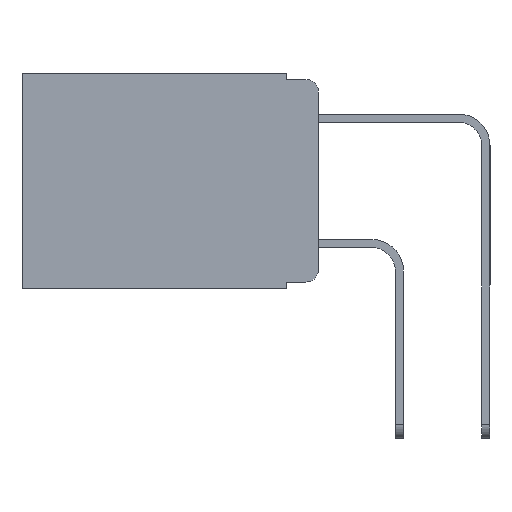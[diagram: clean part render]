
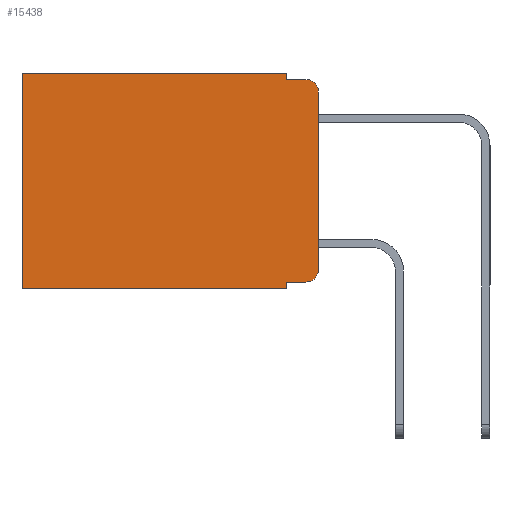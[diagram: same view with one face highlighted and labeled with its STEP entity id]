
A CAD part, left-side view. The second image highlights one B-rep face of the part: STEP entity #15438.
In plain terms, the highlighted planar face has unit normal (-1, 0, 0).
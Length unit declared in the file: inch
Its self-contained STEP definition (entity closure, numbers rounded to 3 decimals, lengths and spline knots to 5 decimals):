
#129 = CARTESIAN_POINT ( 'NONE',  ( 0.298, 0.473, 0. ) ) ;
#816 = VERTEX_POINT ( 'NONE', #3962 ) ;
#822 = DIRECTION ( 'NONE',  ( 0., 1., 0. ) ) ;
#897 = CARTESIAN_POINT ( 'NONE',  ( 0.298, 0., -0.343 ) ) ;
#1227 = ORIENTED_EDGE ( 'NONE', *, *, #1581, .T. ) ;
#1581 = EDGE_CURVE ( 'NONE', #16768, #816, #11439, .T. ) ;
#1775 = VECTOR ( 'NONE', #6155, 39.37008 ) ;
#1896 = VERTEX_POINT ( 'NONE', #14974 ) ;
#2503 = CARTESIAN_POINT ( 'NONE',  ( 0.298, 0.02, -0.03 ) ) ;
#2618 = VECTOR ( 'NONE', #7632, 39.37008 ) ;
#2688 = EDGE_CURVE ( 'NONE', #15392, #16768, #8847, .T. ) ;
#3005 = ORIENTED_EDGE ( 'NONE', *, *, #16992, .T. ) ;
#3034 = DIRECTION ( 'NONE',  ( 0., -1., 0. ) ) ;
#3763 = EDGE_CURVE ( 'NONE', #15392, #4194, #6385, .T. ) ;
#3962 = CARTESIAN_POINT ( 'NONE',  ( 0.298, 0., -0.313 ) ) ;
#3990 = ORIENTED_EDGE ( 'NONE', *, *, #2688, .T. ) ;
#3991 = AXIS2_PLACEMENT_3D ( 'NONE', #16512, #12750, #4978 ) ;
#4094 = DIRECTION ( 'NONE',  ( 0., 0., -1. ) ) ;
#4194 = VERTEX_POINT ( 'NONE', #15497 ) ;
#4494 = LINE ( 'NONE', #129, #5742 ) ;
#4729 = EDGE_CURVE ( 'NONE', #1896, #7967, #4494, .T. ) ;
#4978 = DIRECTION ( 'NONE',  ( 0., 0., -1. ) ) ;
#5184 = AXIS2_PLACEMENT_3D ( 'NONE', #2503, #11911, #4094 ) ;
#5299 = LINE ( 'NONE', #7913, #15559 ) ;
#5421 = DIRECTION ( 'NONE',  ( 0., 0., -1. ) ) ;
#5434 = VECTOR ( 'NONE', #3034, 39.37008 ) ;
#5614 = EDGE_CURVE ( 'NONE', #13787, #12726, #11580, .T. ) ;
#5742 = VECTOR ( 'NONE', #8728, 39.37008 ) ;
#6155 = DIRECTION ( 'NONE',  ( 0., 1., 0. ) ) ;
#6385 = LINE ( 'NONE', #15324, #2618 ) ;
#6475 = EDGE_CURVE ( 'NONE', #12726, #7217, #5299, .T. ) ;
#6719 = ORIENTED_EDGE ( 'NONE', *, *, #5614, .F. ) ;
#6771 = CARTESIAN_POINT ( 'NONE',  ( 0.298, 0.02, -0.313 ) ) ;
#7217 = VERTEX_POINT ( 'NONE', #14213 ) ;
#7240 = DIRECTION ( 'NONE',  ( 0., 0., -1. ) ) ;
#7342 = EDGE_CURVE ( 'NONE', #14983, #7217, #13964, .T. ) ;
#7632 = DIRECTION ( 'NONE',  ( 0., 0., -1. ) ) ;
#7913 = CARTESIAN_POINT ( 'NONE',  ( 0.298, 0.051, -0.01 ) ) ;
#7914 = ORIENTED_EDGE ( 'NONE', *, *, #3763, .F. ) ;
#7967 = VERTEX_POINT ( 'NONE', #10628 ) ;
#8108 = EDGE_LOOP ( 'NONE', ( #8900, #16126, #12771, #6719, #3005, #17295, #10115, #7914, #3990, #1227 ) ) ;
#8112 = CARTESIAN_POINT ( 'NONE',  ( 0.298, 0., -0.03 ) ) ;
#8404 = CARTESIAN_POINT ( 'NONE',  ( 0.298, 0.051, -0.333 ) ) ;
#8728 = DIRECTION ( 'NONE',  ( 0., 0., -1. ) ) ;
#8738 = EDGE_CURVE ( 'NONE', #4194, #7967, #13729, .T. ) ;
#8824 = PLANE ( 'NONE',  #3991 ) ;
#8847 = LINE ( 'NONE', #8404, #5434 ) ;
#8900 = ORIENTED_EDGE ( 'NONE', *, *, #9059, .F. ) ;
#9059 = EDGE_CURVE ( 'NONE', #14983, #816, #16663, .T. ) ;
#10014 = CARTESIAN_POINT ( 'NONE',  ( 0.298, 0.051, -0.333 ) ) ;
#10115 = ORIENTED_EDGE ( 'NONE', *, *, #8738, .F. ) ;
#10628 = CARTESIAN_POINT ( 'NONE',  ( 0.298, 0.473, -0.343 ) ) ;
#10680 = VECTOR ( 'NONE', #822, 39.37008 ) ;
#11319 = CARTESIAN_POINT ( 'NONE',  ( 0.298, 0.051, -0.01 ) ) ;
#11350 = CARTESIAN_POINT ( 'NONE',  ( 0.298, 0., 0. ) ) ;
#11439 = CIRCLE ( 'NONE', #14627, 0.02 ) ;
#11580 = LINE ( 'NONE', #15345, #14593 ) ;
#11803 = CARTESIAN_POINT ( 'NONE',  ( 0.298, 0.051, 0. ) ) ;
#11911 = DIRECTION ( 'NONE',  ( -1., 0., 0. ) ) ;
#12726 = VERTEX_POINT ( 'NONE', #11319 ) ;
#12750 = DIRECTION ( 'NONE',  ( 1., 0., 0. ) ) ;
#12771 = ORIENTED_EDGE ( 'NONE', *, *, #6475, .F. ) ;
#12915 = VECTOR ( 'NONE', #7240, 39.37008 ) ;
#13032 = DIRECTION ( 'NONE',  ( -1., 0., 0. ) ) ;
#13127 = DIRECTION ( 'NONE',  ( 0., -1., 0. ) ) ;
#13729 = LINE ( 'NONE', #897, #10680 ) ;
#13787 = VERTEX_POINT ( 'NONE', #11803 ) ;
#13815 = LINE ( 'NONE', #11350, #1775 ) ;
#13964 = CIRCLE ( 'NONE', #5184, 0.02 ) ;
#14081 = DIRECTION ( 'NONE',  ( 0., 0., -1. ) ) ;
#14213 = CARTESIAN_POINT ( 'NONE',  ( 0.298, 0.02, -0.01 ) ) ;
#14593 = VECTOR ( 'NONE', #14081, 39.37008 ) ;
#14627 = AXIS2_PLACEMENT_3D ( 'NONE', #6771, #13032, #5421 ) ;
#14935 = CARTESIAN_POINT ( 'NONE',  ( 0.298, 0.02, -0.333 ) ) ;
#14974 = CARTESIAN_POINT ( 'NONE',  ( 0.298, 0.473, 0. ) ) ;
#14983 = VERTEX_POINT ( 'NONE', #8112 ) ;
#15033 = FACE_OUTER_BOUND ( 'NONE', #8108, .T. ) ;
#15324 = CARTESIAN_POINT ( 'NONE',  ( 0.298, 0.051, 0. ) ) ;
#15345 = CARTESIAN_POINT ( 'NONE',  ( 0.298, 0.051, 0. ) ) ;
#15392 = VERTEX_POINT ( 'NONE', #10014 ) ;
#15438 = ADVANCED_FACE ( 'NONE', ( #15033 ), #8824, .F. ) ;
#15497 = CARTESIAN_POINT ( 'NONE',  ( 0.298, 0.051, -0.343 ) ) ;
#15559 = VECTOR ( 'NONE', #13127, 39.37008 ) ;
#16126 = ORIENTED_EDGE ( 'NONE', *, *, #7342, .T. ) ;
#16512 = CARTESIAN_POINT ( 'NONE',  ( 0.298, 0., 0. ) ) ;
#16663 = LINE ( 'NONE', #17445, #12915 ) ;
#16768 = VERTEX_POINT ( 'NONE', #14935 ) ;
#16992 = EDGE_CURVE ( 'NONE', #13787, #1896, #13815, .T. ) ;
#17295 = ORIENTED_EDGE ( 'NONE', *, *, #4729, .T. ) ;
#17445 = CARTESIAN_POINT ( 'NONE',  ( 0.298, 0., 0. ) ) ;
